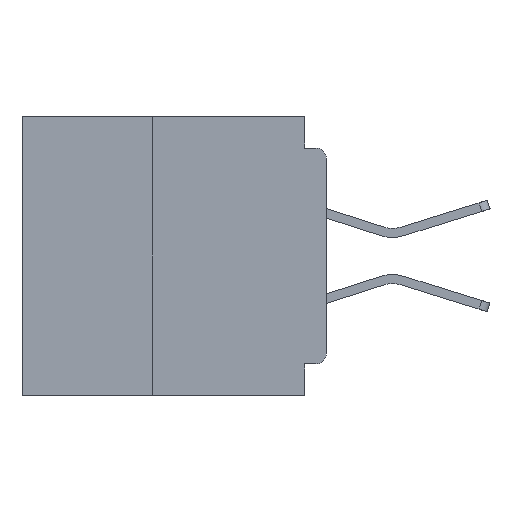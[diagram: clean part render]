
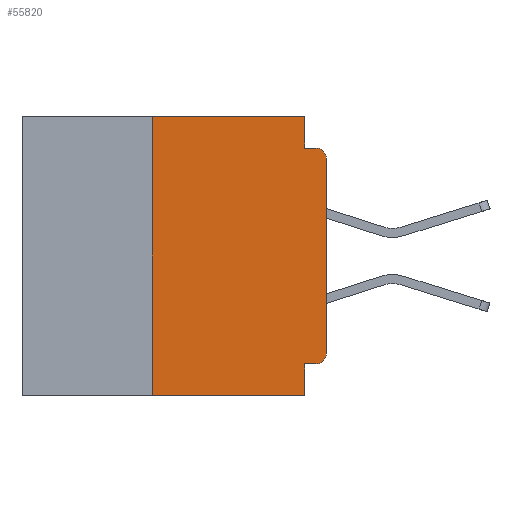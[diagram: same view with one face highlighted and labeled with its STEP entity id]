
A CAD part, left-side view. The second image highlights one B-rep face of the part: STEP entity #55820.
In plain terms, the highlighted planar face has unit normal (-1, 0, 0).
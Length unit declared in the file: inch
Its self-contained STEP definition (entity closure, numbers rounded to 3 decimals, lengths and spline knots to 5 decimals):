
#452 = VERTEX_POINT ( 'NONE', #29019 ) ;
#1449 = DIRECTION ( 'NONE',  ( 0., 0., 1. ) ) ;
#1576 = VECTOR ( 'NONE', #4960, 39.37008 ) ;
#1734 = ORIENTED_EDGE ( 'NONE', *, *, #25945, .T. ) ;
#2042 = CARTESIAN_POINT ( 'NONE',  ( 0., 0., 0. ) ) ;
#2153 = DIRECTION ( 'NONE',  ( 0., 0., -1. ) ) ;
#2229 = DIRECTION ( 'NONE',  ( 0., 0., -1. ) ) ;
#2853 = CARTESIAN_POINT ( 'NONE',  ( 0., 0.25, 0. ) ) ;
#4960 = DIRECTION ( 'NONE',  ( 0., 0., -1. ) ) ;
#5366 = VERTEX_POINT ( 'NONE', #26088 ) ;
#5616 = EDGE_CURVE ( 'NONE', #452, #56125, #52366, .T. ) ;
#5933 = CARTESIAN_POINT ( 'NONE',  ( 0., 0.031, -0.4 ) ) ;
#6407 = CARTESIAN_POINT ( 'NONE',  ( 0., 0.031, 0. ) ) ;
#6461 = CARTESIAN_POINT ( 'NONE',  ( 0., 0., -0.045 ) ) ;
#6462 = ORIENTED_EDGE ( 'NONE', *, *, #34403, .T. ) ;
#6788 = ORIENTED_EDGE ( 'NONE', *, *, #49296, .T. ) ;
#6807 = CARTESIAN_POINT ( 'NONE',  ( 0., 0.437, 0. ) ) ;
#9350 = VECTOR ( 'NONE', #54822, 39.37008 ) ;
#9768 = ORIENTED_EDGE ( 'NONE', *, *, #27325, .F. ) ;
#10723 = LINE ( 'NONE', #6807, #9350 ) ;
#11708 = LINE ( 'NONE', #2042, #30938 ) ;
#13278 = LINE ( 'NONE', #27039, #1576 ) ;
#13784 = VERTEX_POINT ( 'NONE', #51124 ) ;
#13836 = CARTESIAN_POINT ( 'NONE',  ( 0., 0.437, 0. ) ) ;
#14811 = CARTESIAN_POINT ( 'NONE',  ( 0., 0.031, -0.355 ) ) ;
#15924 = ORIENTED_EDGE ( 'NONE', *, *, #47709, .T. ) ;
#18246 = DIRECTION ( 'NONE',  ( 0., 0., -1. ) ) ;
#18632 = VERTEX_POINT ( 'NONE', #54806 ) ;
#19717 = CARTESIAN_POINT ( 'NONE',  ( 0., 0., -0.355 ) ) ;
#19859 = EDGE_LOOP ( 'NONE', ( #6462, #6788, #29419, #30036, #55393, #41819, #15924, #9768, #53156, #1734 ) ) ;
#20538 = EDGE_CURVE ( 'NONE', #56125, #54970, #10723, .T. ) ;
#20836 = EDGE_CURVE ( 'NONE', #5366, #18632, #39448, .T. ) ;
#21150 = VECTOR ( 'NONE', #30624, 39.37008 ) ;
#23291 = EDGE_CURVE ( 'NONE', #54970, #5366, #56236, .T. ) ;
#23919 = VERTEX_POINT ( 'NONE', #5933 ) ;
#24352 = CARTESIAN_POINT ( 'NONE',  ( 0., 0.015, -0.34 ) ) ;
#25945 = EDGE_CURVE ( 'NONE', #28756, #13784, #51017, .T. ) ;
#26088 = CARTESIAN_POINT ( 'NONE',  ( 0., 0.031, -0.045 ) ) ;
#26228 = CARTESIAN_POINT ( 'NONE',  ( 0., 0.437, -0.4 ) ) ;
#27039 = CARTESIAN_POINT ( 'NONE',  ( 0., 0.031, -0.4 ) ) ;
#27325 = EDGE_CURVE ( 'NONE', #46338, #23919, #13278, .T. ) ;
#27866 = CARTESIAN_POINT ( 'NONE',  ( 0., 0.015, -0.355 ) ) ;
#28542 = DIRECTION ( 'NONE',  ( 0., 1., 0. ) ) ;
#28556 = DIRECTION ( 'NONE',  ( -1., 0., 0. ) ) ;
#28701 = LINE ( 'NONE', #26228, #21150 ) ;
#28756 = VERTEX_POINT ( 'NONE', #27866 ) ;
#28757 = DIRECTION ( 'NONE',  ( 0., 0., -1. ) ) ;
#29019 = CARTESIAN_POINT ( 'NONE',  ( 0., 0.25, -0.4 ) ) ;
#29419 = ORIENTED_EDGE ( 'NONE', *, *, #20836, .F. ) ;
#30036 = ORIENTED_EDGE ( 'NONE', *, *, #23291, .F. ) ;
#30071 = VECTOR ( 'NONE', #28542, 39.37008 ) ;
#30624 = DIRECTION ( 'NONE',  ( 0., -1., 0. ) ) ;
#30938 = VECTOR ( 'NONE', #37115, 39.37008 ) ;
#31264 = FACE_OUTER_BOUND ( 'NONE', #19859, .T. ) ;
#31288 = PLANE ( 'NONE',  #32464 ) ;
#32464 = AXIS2_PLACEMENT_3D ( 'NONE', #13836, #44415, #18246 ) ;
#32722 = DIRECTION ( 'NONE',  ( 0., -1., 0. ) ) ;
#34403 = EDGE_CURVE ( 'NONE', #13784, #51960, #11708, .T. ) ;
#36133 = CARTESIAN_POINT ( 'NONE',  ( 0., 0.031, 0. ) ) ;
#36557 = EDGE_CURVE ( 'NONE', #28756, #46338, #41657, .T. ) ;
#37115 = DIRECTION ( 'NONE',  ( 0., 0., 1. ) ) ;
#39384 = CIRCLE ( 'NONE', #41728, 0.015 ) ;
#39446 = CARTESIAN_POINT ( 'NONE',  ( 0., 0., -0.06 ) ) ;
#39448 = LINE ( 'NONE', #6461, #49662 ) ;
#40797 = VECTOR ( 'NONE', #1449, 39.37008 ) ;
#41657 = LINE ( 'NONE', #19717, #30071 ) ;
#41728 = AXIS2_PLACEMENT_3D ( 'NONE', #54657, #28556, #2229 ) ;
#41819 = ORIENTED_EDGE ( 'NONE', *, *, #5616, .F. ) ;
#44415 = DIRECTION ( 'NONE',  ( 1., 0., 0. ) ) ;
#44604 = VECTOR ( 'NONE', #2153, 39.37008 ) ;
#46338 = VERTEX_POINT ( 'NONE', #14811 ) ;
#47709 = EDGE_CURVE ( 'NONE', #452, #23919, #28701, .T. ) ;
#49285 = CARTESIAN_POINT ( 'NONE',  ( 0., 0.25, -0.4 ) ) ;
#49296 = EDGE_CURVE ( 'NONE', #51960, #18632, #39384, .T. ) ;
#49662 = VECTOR ( 'NONE', #32722, 39.37008 ) ;
#51017 = CIRCLE ( 'NONE', #56095, 0.015 ) ;
#51124 = CARTESIAN_POINT ( 'NONE',  ( 0., 0., -0.34 ) ) ;
#51960 = VERTEX_POINT ( 'NONE', #39446 ) ;
#52366 = LINE ( 'NONE', #49285, #40797 ) ;
#53156 = ORIENTED_EDGE ( 'NONE', *, *, #36557, .F. ) ;
#54657 = CARTESIAN_POINT ( 'NONE',  ( 0., 0.015, -0.06 ) ) ;
#54806 = CARTESIAN_POINT ( 'NONE',  ( 0., 0.015, -0.045 ) ) ;
#54822 = DIRECTION ( 'NONE',  ( 0., -1., 0. ) ) ;
#54871 = DIRECTION ( 'NONE',  ( -1., 0., 0. ) ) ;
#54970 = VERTEX_POINT ( 'NONE', #36133 ) ;
#55393 = ORIENTED_EDGE ( 'NONE', *, *, #20538, .F. ) ;
#55820 = ADVANCED_FACE ( 'NONE', ( #31264 ), #31288, .F. ) ;
#56095 = AXIS2_PLACEMENT_3D ( 'NONE', #24352, #54871, #28757 ) ;
#56125 = VERTEX_POINT ( 'NONE', #2853 ) ;
#56236 = LINE ( 'NONE', #6407, #44604 ) ;
